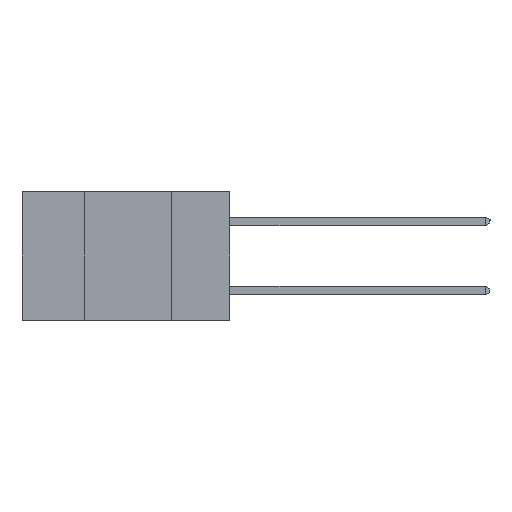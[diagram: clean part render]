
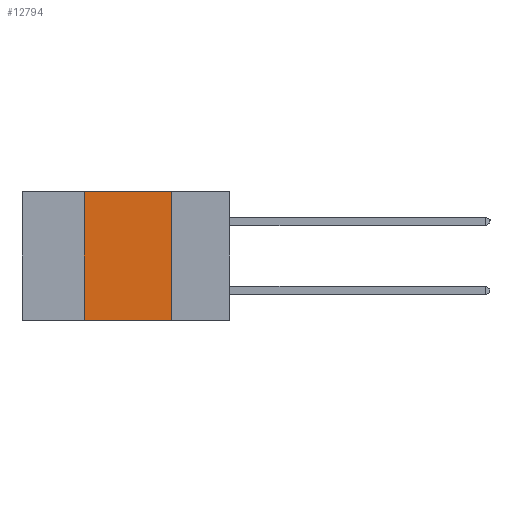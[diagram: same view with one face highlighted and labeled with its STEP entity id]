
A CAD part, left-side view. The second image highlights one B-rep face of the part: STEP entity #12794.
In plain terms, the highlighted planar face has unit normal (-1, 0, 0).
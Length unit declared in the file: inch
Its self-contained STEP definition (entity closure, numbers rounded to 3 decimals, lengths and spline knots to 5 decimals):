
#54 = CARTESIAN_POINT ( 'NONE',  ( 0., 0.42, 0. ) ) ;
#138 = LINE ( 'NONE', #9507, #14803 ) ;
#237 = LINE ( 'NONE', #4384, #13334 ) ;
#948 = ORIENTED_EDGE ( 'NONE', *, *, #11025, .F. ) ;
#2078 = CARTESIAN_POINT ( 'NONE',  ( 0., 0.6, -0.37 ) ) ;
#2504 = EDGE_CURVE ( 'NONE', #13124, #3204, #4442, .T. ) ;
#2723 = CARTESIAN_POINT ( 'NONE',  ( 0., 0.42, -0.37 ) ) ;
#3204 = VERTEX_POINT ( 'NONE', #3583 ) ;
#3311 = CARTESIAN_POINT ( 'NONE',  ( 0., 0.17, 0. ) ) ;
#3534 = AXIS2_PLACEMENT_3D ( 'NONE', #6709, #13778, #15012 ) ;
#3583 = CARTESIAN_POINT ( 'NONE',  ( 0., 0.17, -0.37 ) ) ;
#4384 = CARTESIAN_POINT ( 'NONE',  ( 0., 0.42, -0.37 ) ) ;
#4442 = LINE ( 'NONE', #2078, #9706 ) ;
#4723 = EDGE_CURVE ( 'NONE', #13124, #11361, #237, .T. ) ;
#4833 = LINE ( 'NONE', #14048, #13833 ) ;
#6709 = CARTESIAN_POINT ( 'NONE',  ( 0., 0.6, 0. ) ) ;
#7283 = EDGE_LOOP ( 'NONE', ( #7528, #948, #14547, #8323 ) ) ;
#7528 = ORIENTED_EDGE ( 'NONE', *, *, #11528, .F. ) ;
#8323 = ORIENTED_EDGE ( 'NONE', *, *, #2504, .T. ) ;
#8759 = VERTEX_POINT ( 'NONE', #3311 ) ;
#9507 = CARTESIAN_POINT ( 'NONE',  ( 0., 0.17, -0.37 ) ) ;
#9706 = VECTOR ( 'NONE', #10360, 39.37008 ) ;
#10360 = DIRECTION ( 'NONE',  ( 0., -1., 0. ) ) ;
#11025 = EDGE_CURVE ( 'NONE', #11361, #8759, #4833, .T. ) ;
#11361 = VERTEX_POINT ( 'NONE', #54 ) ;
#11528 = EDGE_CURVE ( 'NONE', #8759, #3204, #138, .T. ) ;
#11598 = DIRECTION ( 'NONE',  ( 0., -1., 0. ) ) ;
#12645 = PLANE ( 'NONE',  #3534 ) ;
#12794 = ADVANCED_FACE ( 'NONE', ( #14800 ), #12645, .F. ) ;
#13124 = VERTEX_POINT ( 'NONE', #2723 ) ;
#13334 = VECTOR ( 'NONE', #14688, 39.37008 ) ;
#13778 = DIRECTION ( 'NONE',  ( 1., 0., 0. ) ) ;
#13833 = VECTOR ( 'NONE', #11598, 39.37008 ) ;
#14048 = CARTESIAN_POINT ( 'NONE',  ( 0., 0.6, 0. ) ) ;
#14348 = DIRECTION ( 'NONE',  ( 0., 0., -1. ) ) ;
#14547 = ORIENTED_EDGE ( 'NONE', *, *, #4723, .F. ) ;
#14688 = DIRECTION ( 'NONE',  ( 0., 0., 1. ) ) ;
#14800 = FACE_OUTER_BOUND ( 'NONE', #7283, .T. ) ;
#14803 = VECTOR ( 'NONE', #14348, 39.37008 ) ;
#15012 = DIRECTION ( 'NONE',  ( 0., 0., -1. ) ) ;
